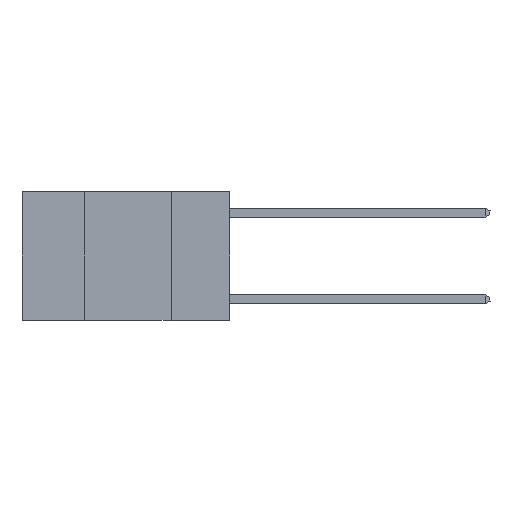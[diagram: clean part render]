
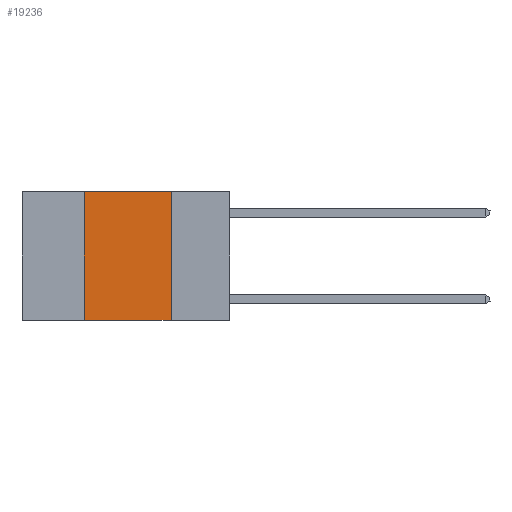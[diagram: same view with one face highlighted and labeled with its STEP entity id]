
A CAD part, left-side view. The second image highlights one B-rep face of the part: STEP entity #19236.
In plain terms, the highlighted planar face has unit normal (-1, 0, 0).
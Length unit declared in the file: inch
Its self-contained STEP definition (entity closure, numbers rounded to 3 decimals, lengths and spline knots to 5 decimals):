
#246 = VERTEX_POINT ( 'NONE', #6477 ) ;
#351 = ORIENTED_EDGE ( 'NONE', *, *, #16967, .T. ) ;
#1842 = ORIENTED_EDGE ( 'NONE', *, *, #26016, .F. ) ;
#2338 = DIRECTION ( 'NONE',  ( 0., 0., 1. ) ) ;
#3896 = VECTOR ( 'NONE', #15216, 39.37008 ) ;
#4797 = LINE ( 'NONE', #16692, #22263 ) ;
#4825 = ORIENTED_EDGE ( 'NONE', *, *, #13544, .F. ) ;
#6039 = DIRECTION ( 'NONE',  ( 1., 0., 0. ) ) ;
#6477 = CARTESIAN_POINT ( 'NONE',  ( 0., 0.42, 0. ) ) ;
#6537 = VECTOR ( 'NONE', #15213, 39.37008 ) ;
#8351 = PLANE ( 'NONE',  #14028 ) ;
#8631 = EDGE_CURVE ( 'NONE', #246, #12509, #25459, .T. ) ;
#12462 = DIRECTION ( 'NONE',  ( 0., 0., -1. ) ) ;
#12509 = VERTEX_POINT ( 'NONE', #23649 ) ;
#13544 = EDGE_CURVE ( 'NONE', #12509, #16725, #27064, .T. ) ;
#14028 = AXIS2_PLACEMENT_3D ( 'NONE', #29652, #6039, #22653 ) ;
#15213 = DIRECTION ( 'NONE',  ( 0., -1., 0. ) ) ;
#15216 = DIRECTION ( 'NONE',  ( 0., -1., 0. ) ) ;
#16692 = CARTESIAN_POINT ( 'NONE',  ( 0., 0.42, 0. ) ) ;
#16725 = VERTEX_POINT ( 'NONE', #21036 ) ;
#16967 = EDGE_CURVE ( 'NONE', #30628, #16725, #22840, .T. ) ;
#19236 = ADVANCED_FACE ( 'NONE', ( #24191 ), #8351, .F. ) ;
#19567 = CARTESIAN_POINT ( 'NONE',  ( 0., 0.42, -0.37 ) ) ;
#21036 = CARTESIAN_POINT ( 'NONE',  ( 0., 0.17, -0.37 ) ) ;
#21553 = VECTOR ( 'NONE', #12462, 39.37008 ) ;
#22263 = VECTOR ( 'NONE', #2338, 39.37008 ) ;
#22653 = DIRECTION ( 'NONE',  ( 0., 0., -1. ) ) ;
#22840 = LINE ( 'NONE', #29352, #3896 ) ;
#23019 = ORIENTED_EDGE ( 'NONE', *, *, #8631, .F. ) ;
#23649 = CARTESIAN_POINT ( 'NONE',  ( 0., 0.17, 0. ) ) ;
#24191 = FACE_OUTER_BOUND ( 'NONE', #28967, .T. ) ;
#25459 = LINE ( 'NONE', #27094, #6537 ) ;
#26016 = EDGE_CURVE ( 'NONE', #30628, #246, #4797, .T. ) ;
#26627 = CARTESIAN_POINT ( 'NONE',  ( 0., 0.17, 0. ) ) ;
#27064 = LINE ( 'NONE', #26627, #21553 ) ;
#27094 = CARTESIAN_POINT ( 'NONE',  ( 0., 0.6, 0. ) ) ;
#28967 = EDGE_LOOP ( 'NONE', ( #4825, #23019, #1842, #351 ) ) ;
#29352 = CARTESIAN_POINT ( 'NONE',  ( 0., 0.6, -0.37 ) ) ;
#29652 = CARTESIAN_POINT ( 'NONE',  ( 0., 0.6, 0. ) ) ;
#30628 = VERTEX_POINT ( 'NONE', #19567 ) ;
